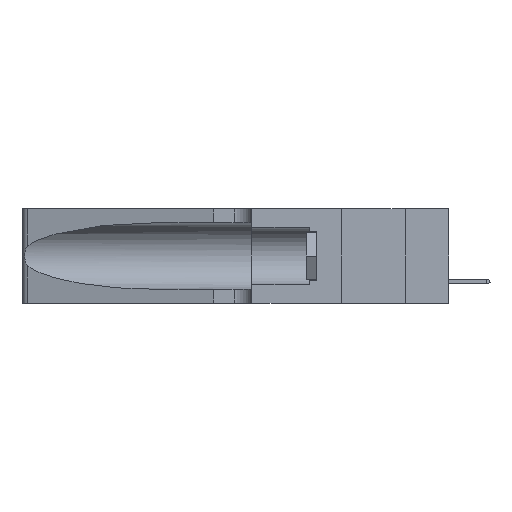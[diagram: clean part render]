
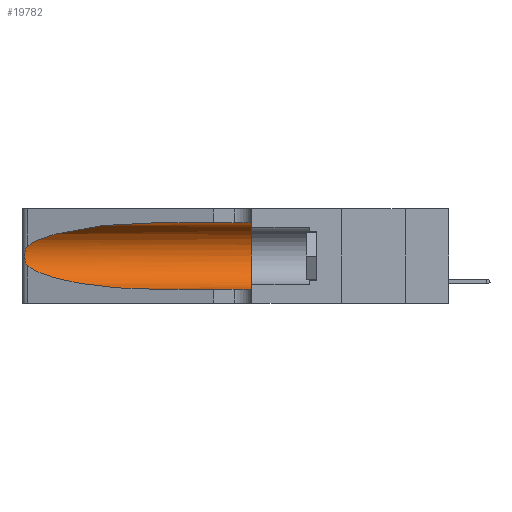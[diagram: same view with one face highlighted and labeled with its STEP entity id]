
A CAD part, left-side view. The second image highlights one B-rep face of the part: STEP entity #19782.
In plain terms, the highlighted cylindrical face has radius 3.308 mm (diameter 6.617 mm), a partial arc.
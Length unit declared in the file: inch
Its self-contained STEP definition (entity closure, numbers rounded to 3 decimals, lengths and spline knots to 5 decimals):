
#73 = CARTESIAN_POINT ( 'NONE',  ( 0.25487, 1.22718, 0.14631 ) ) ;
#194 = LINE ( 'NONE', #2368, #21628 ) ;
#566 = CARTESIAN_POINT ( 'NONE',  ( 0.1305, 1.61858, 0.185 ) ) ;
#1485 = CARTESIAN_POINT ( 'NONE',  ( 0.18966, 0.96281, 0.05475 ) ) ;
#1578 = EDGE_CURVE ( 'NONE', #14939, #4421, #8344, .T. ) ;
#1909 = CARTESIAN_POINT ( 'NONE',  ( 0.1305, 0.72297, 0.05475 ) ) ;
#2243 = DIRECTION ( 'NONE',  ( 0., 0., -1. ) ) ;
#2368 = CARTESIAN_POINT ( 'NONE',  ( 0.1305, 1.61858, 0.05475 ) ) ;
#2376 = CARTESIAN_POINT ( 'NONE',  ( 0.25487, 1.22718, 0.22369 ) ) ;
#2866 = B_SPLINE_CURVE_WITH_KNOTS ( 'NONE', 3,
 ( #2376, #10710, #11794, #11868, #14868, #6568, #18277, #8230, #9608, #11406, #13095, #11764, #3403, #6775 ),
 .UNSPECIFIED., .F., .F.,
 ( 4, 2, 2, 2, 2, 2, 4 ),
 ( 0., 0.00027, 0.00053, 0.00107, 0.0016, 0.00187, 0.00214 ),
 .UNSPECIFIED. ) ;
#3403 = CARTESIAN_POINT ( 'NONE',  ( 0.25555, 1.22993, 0.14849 ) ) ;
#3575 = CARTESIAN_POINT ( 'NONE',  ( 0.25487, 1.22718, 0.22369 ) ) ;
#3780 = VERTEX_POINT ( 'NONE', #3575 ) ;
#4378 = EDGE_CURVE ( 'NONE', #18933, #7057, #5765, .T. ) ;
#4421 = VERTEX_POINT ( 'NONE', #18390 ) ;
#4510 = CARTESIAN_POINT ( 'NONE',  ( 0.1305, 0.72297, 0.31525 ) ) ;
#4780 = AXIS2_PLACEMENT_3D ( 'NONE', #566, #12219, #2243 ) ;
#5099 = CARTESIAN_POINT ( 'NONE',  ( 0.2373, 1.15595, 0.08982 ) ) ;
#5676 = CARTESIAN_POINT ( 'NONE',  ( 0.25487, 1.22718, 0.22369 ) ) ;
#5765 =( BOUNDED_CURVE ( )  B_SPLINE_CURVE ( 3, ( #73, #5099, #1485, #1909 ),
 .UNSPECIFIED., .F., .T. ) 
 B_SPLINE_CURVE_WITH_KNOTS ( ( 4, 4 ),
 ( 3.44316, 4.71239 ),
 .UNSPECIFIED. ) 
 CURVE ( )  GEOMETRIC_REPRESENTATION_ITEM ( )  RATIONAL_B_SPLINE_CURVE ( ( 1., 0.87, 0.87, 1. ) ) 
 REPRESENTATION_ITEM ( '' )  );
#5890 = DIRECTION ( 'NONE',  ( 0., 0., 1. ) ) ;
#6385 = EDGE_CURVE ( 'NONE', #3780, #18933, #2866, .T. ) ;
#6406 = FACE_OUTER_BOUND ( 'NONE', #12258, .T. ) ;
#6568 = CARTESIAN_POINT ( 'NONE',  ( 0.26018, 1.23835, 0.19895 ) ) ;
#6775 = CARTESIAN_POINT ( 'NONE',  ( 0.25487, 1.22718, 0.14631 ) ) ;
#7057 = VERTEX_POINT ( 'NONE', #15948 ) ;
#7213 = CIRCLE ( 'NONE', #20019, 0.13025 ) ;
#7985 = CARTESIAN_POINT ( 'NONE',  ( 0.25487, 1.22718, 0.14631 ) ) ;
#8230 = CARTESIAN_POINT ( 'NONE',  ( 0.26075, 1.23896, 0.178 ) ) ;
#8344 = LINE ( 'NONE', #11820, #14401 ) ;
#9012 = DIRECTION ( 'NONE',  ( 0., -1., 0. ) ) ;
#9608 = CARTESIAN_POINT ( 'NONE',  ( 0.26017, 1.23833, 0.17102 ) ) ;
#10268 =( BOUNDED_CURVE ( )  B_SPLINE_CURVE ( 3, ( #18975, #15825, #17419, #5676 ),
 .UNSPECIFIED., .F., .F. ) 
 B_SPLINE_CURVE_WITH_KNOTS ( ( 4, 4 ),
 ( 1.5708, 2.84003 ),
 .UNSPECIFIED. ) 
 CURVE ( )  GEOMETRIC_REPRESENTATION_ITEM ( )  RATIONAL_B_SPLINE_CURVE ( ( 1., 0.87, 0.87, 1. ) ) 
 REPRESENTATION_ITEM ( '' )  );
#10518 = ORIENTED_EDGE ( 'NONE', *, *, #14727, .T. ) ;
#10710 = CARTESIAN_POINT ( 'NONE',  ( 0.25555, 1.22994, 0.2215 ) ) ;
#11406 = CARTESIAN_POINT ( 'NONE',  ( 0.25856, 1.23593, 0.16098 ) ) ;
#11721 = VERTEX_POINT ( 'NONE', #20795 ) ;
#11764 = CARTESIAN_POINT ( 'NONE',  ( 0.25639, 1.23186, 0.15144 ) ) ;
#11794 = CARTESIAN_POINT ( 'NONE',  ( 0.25639, 1.23184, 0.21858 ) ) ;
#11820 = CARTESIAN_POINT ( 'NONE',  ( 0.1305, 1.61858, 0.31525 ) ) ;
#11868 = CARTESIAN_POINT ( 'NONE',  ( 0.25787, 1.23484, 0.2124 ) ) ;
#12219 = DIRECTION ( 'NONE',  ( 0., -1., 0. ) ) ;
#12258 = EDGE_LOOP ( 'NONE', ( #10518, #18737, #20123, #17496, #14123, #12732 ) ) ;
#12540 = CARTESIAN_POINT ( 'NONE',  ( 0.1305, 0.35, 0.185 ) ) ;
#12732 = ORIENTED_EDGE ( 'NONE', *, *, #1578, .F. ) ;
#13095 = CARTESIAN_POINT ( 'NONE',  ( 0.25789, 1.23486, 0.15765 ) ) ;
#13566 = DIRECTION ( 'NONE',  ( 0., -1., 0. ) ) ;
#14123 = ORIENTED_EDGE ( 'NONE', *, *, #17563, .F. ) ;
#14401 = VECTOR ( 'NONE', #13566, 39.37008 ) ;
#14727 = EDGE_CURVE ( 'NONE', #14939, #3780, #10268, .T. ) ;
#14868 = CARTESIAN_POINT ( 'NONE',  ( 0.25854, 1.2359, 0.20912 ) ) ;
#14939 = VERTEX_POINT ( 'NONE', #4510 ) ;
#15825 = CARTESIAN_POINT ( 'NONE',  ( 0.18966, 0.96281, 0.31525 ) ) ;
#15948 = CARTESIAN_POINT ( 'NONE',  ( 0.1305, 0.72297, 0.05475 ) ) ;
#17416 = DIRECTION ( 'NONE',  ( 0., 1., 0. ) ) ;
#17419 = CARTESIAN_POINT ( 'NONE',  ( 0.2373, 1.15595, 0.28018 ) ) ;
#17496 = ORIENTED_EDGE ( 'NONE', *, *, #18576, .T. ) ;
#17563 = EDGE_CURVE ( 'NONE', #4421, #11721, #7213, .T. ) ;
#18277 = CARTESIAN_POINT ( 'NONE',  ( 0.26075, 1.23896, 0.19203 ) ) ;
#18390 = CARTESIAN_POINT ( 'NONE',  ( 0.1305, 0.35, 0.31525 ) ) ;
#18576 = EDGE_CURVE ( 'NONE', #7057, #11721, #194, .T. ) ;
#18737 = ORIENTED_EDGE ( 'NONE', *, *, #6385, .T. ) ;
#18933 = VERTEX_POINT ( 'NONE', #7985 ) ;
#18975 = CARTESIAN_POINT ( 'NONE',  ( 0.1305, 0.72297, 0.31525 ) ) ;
#19227 = CYLINDRICAL_SURFACE ( 'NONE', #4780, 0.13025 ) ;
#19782 = ADVANCED_FACE ( 'NONE', ( #6406 ), #19227, .F. ) ;
#20019 = AXIS2_PLACEMENT_3D ( 'NONE', #12540, #17416, #5890 ) ;
#20123 = ORIENTED_EDGE ( 'NONE', *, *, #4378, .T. ) ;
#20795 = CARTESIAN_POINT ( 'NONE',  ( 0.1305, 0.35, 0.05475 ) ) ;
#21628 = VECTOR ( 'NONE', #9012, 39.37008 ) ;
